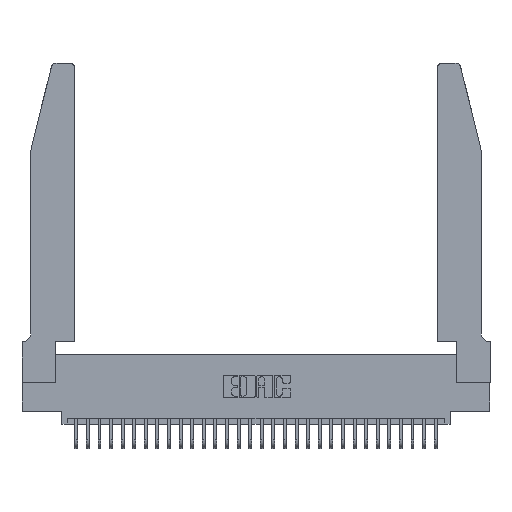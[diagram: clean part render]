
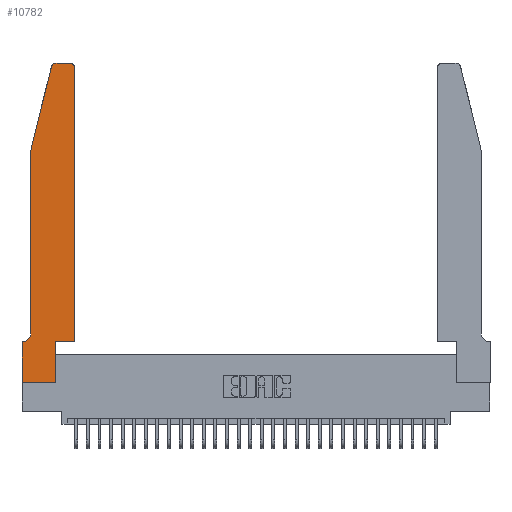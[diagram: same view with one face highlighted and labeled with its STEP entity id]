
A CAD part, top view. The second image highlights one B-rep face of the part: STEP entity #10782.
In plain terms, the highlighted planar face has unit normal (0, 0, 1).
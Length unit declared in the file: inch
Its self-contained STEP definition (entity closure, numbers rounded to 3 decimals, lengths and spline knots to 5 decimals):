
#184 = EDGE_CURVE ( 'NONE', #10911, #10960, #1109, .T. ) ;
#239 = VECTOR ( 'NONE', #18105, 39.37008 ) ;
#500 = CARTESIAN_POINT ( 'NONE',  ( 0.284, 2.75, 0.37 ) ) ;
#1109 = CIRCLE ( 'NONE', #26947, 0.07 ) ;
#1132 = CIRCLE ( 'NONE', #14062, 0.03 ) ;
#1803 = VERTEX_POINT ( 'NONE', #9535 ) ;
#2464 = VECTOR ( 'NONE', #32815, 39.37008 ) ;
#2518 = DIRECTION ( 'NONE',  ( 1., 0., 0. ) ) ;
#2710 = CARTESIAN_POINT ( 'NONE',  ( 0.4505, 0.35, 0.37 ) ) ;
#2935 = ORIENTED_EDGE ( 'NONE', *, *, #15527, .T. ) ;
#3083 = CIRCLE ( 'NONE', #22359, 0.03 ) ;
#3107 = VECTOR ( 'NONE', #7355, 39.37008 ) ;
#3114 = CARTESIAN_POINT ( 'NONE',  ( 0.0755, 0.35, 0.37 ) ) ;
#3702 = VERTEX_POINT ( 'NONE', #31811 ) ;
#4376 = ORIENTED_EDGE ( 'NONE', *, *, #26574, .T. ) ;
#4494 = VERTEX_POINT ( 'NONE', #19163 ) ;
#4568 = CARTESIAN_POINT ( 'NONE',  ( 0.0755, 2., 0.37 ) ) ;
#4871 = CARTESIAN_POINT ( 'NONE',  ( 0., 0., 0.37 ) ) ;
#4957 = CARTESIAN_POINT ( 'NONE',  ( 0.25487, 2.72718, 0.37 ) ) ;
#5204 = CARTESIAN_POINT ( 'NONE',  ( 0., 0.35, 0.37 ) ) ;
#5278 = DIRECTION ( 'NONE',  ( 0., 1., 0. ) ) ;
#5497 = DIRECTION ( 'NONE',  ( 0., 0., 1. ) ) ;
#5579 = ORIENTED_EDGE ( 'NONE', *, *, #6505, .T. ) ;
#6347 = DIRECTION ( 'NONE',  ( 1., 0., 0. ) ) ;
#6505 = EDGE_CURVE ( 'NONE', #4494, #7842, #20833, .T. ) ;
#6745 = EDGE_CURVE ( 'NONE', #9072, #10911, #13109, .T. ) ;
#7355 = DIRECTION ( 'NONE',  ( 1., 0., 0. ) ) ;
#7842 = VERTEX_POINT ( 'NONE', #19336 ) ;
#7913 = DIRECTION ( 'NONE',  ( 1., 0., 0. ) ) ;
#8019 = ORIENTED_EDGE ( 'NONE', *, *, #24753, .T. ) ;
#8052 = FACE_OUTER_BOUND ( 'NONE', #30361, .T. ) ;
#8519 = CARTESIAN_POINT ( 'NONE',  ( 0.0055, 0.35, 0.37 ) ) ;
#8548 = VERTEX_POINT ( 'NONE', #12256 ) ;
#9049 = ORIENTED_EDGE ( 'NONE', *, *, #23664, .T. ) ;
#9072 = VERTEX_POINT ( 'NONE', #14395 ) ;
#9352 = CARTESIAN_POINT ( 'NONE',  ( 0.0055, 0.42, 0.37 ) ) ;
#9535 = CARTESIAN_POINT ( 'NONE',  ( 0.4205, 2.75, 0.37 ) ) ;
#10027 = VECTOR ( 'NONE', #5278, 39.37008 ) ;
#10782 = ADVANCED_FACE ( 'NONE', ( #8052 ), #18148, .T. ) ;
#10911 = VERTEX_POINT ( 'NONE', #11079 ) ;
#10960 = VERTEX_POINT ( 'NONE', #8519 ) ;
#11079 = CARTESIAN_POINT ( 'NONE',  ( 0.0755, 0.42, 0.37 ) ) ;
#11301 = LINE ( 'NONE', #4568, #13681 ) ;
#11766 = CARTESIAN_POINT ( 'NONE',  ( 0.2865, 0.35, 0.37 ) ) ;
#12148 = DIRECTION ( 'NONE',  ( 0., 0., -1. ) ) ;
#12256 = CARTESIAN_POINT ( 'NONE',  ( 0.4505, 2.72, 0.37 ) ) ;
#12583 = LINE ( 'NONE', #27706, #16585 ) ;
#12739 = CARTESIAN_POINT ( 'NONE',  ( 0., 0., 0.37 ) ) ;
#13109 = LINE ( 'NONE', #29508, #22252 ) ;
#13526 = DIRECTION ( 'NONE',  ( 1., 0., 0. ) ) ;
#13681 = VECTOR ( 'NONE', #27495, 39.37008 ) ;
#14062 = AXIS2_PLACEMENT_3D ( 'NONE', #18311, #5497, #13526 ) ;
#14395 = CARTESIAN_POINT ( 'NONE',  ( 0.0755, 2., 0.37 ) ) ;
#15309 = VERTEX_POINT ( 'NONE', #25043 ) ;
#15527 = EDGE_CURVE ( 'NONE', #24561, #9072, #11301, .T. ) ;
#15559 = DIRECTION ( 'NONE',  ( -1., 0., 0. ) ) ;
#16585 = VECTOR ( 'NONE', #2518, 39.37008 ) ;
#16905 = ORIENTED_EDGE ( 'NONE', *, *, #6745, .T. ) ;
#17367 = DIRECTION ( 'NONE',  ( -1., 0., 0. ) ) ;
#17601 = VERTEX_POINT ( 'NONE', #12739 ) ;
#18105 = DIRECTION ( 'NONE',  ( -1., 0., 0. ) ) ;
#18148 = PLANE ( 'NONE',  #27326 ) ;
#18311 = CARTESIAN_POINT ( 'NONE',  ( 0.284, 2.72, 0.37 ) ) ;
#18360 = LINE ( 'NONE', #2710, #10027 ) ;
#18385 = DIRECTION ( 'NONE',  ( 0., -1., 0. ) ) ;
#19163 = CARTESIAN_POINT ( 'NONE',  ( 0.2865, 0., 0.37 ) ) ;
#19336 = CARTESIAN_POINT ( 'NONE',  ( 0.2865, 0.35, 0.37 ) ) ;
#19370 = ORIENTED_EDGE ( 'NONE', *, *, #31069, .T. ) ;
#20011 = VECTOR ( 'NONE', #15559, 39.37008 ) ;
#20019 = VECTOR ( 'NONE', #24338, 39.37008 ) ;
#20102 = ORIENTED_EDGE ( 'NONE', *, *, #184, .T. ) ;
#20575 = CARTESIAN_POINT ( 'NONE',  ( 0.2605, 2.75, 0.37 ) ) ;
#20833 = LINE ( 'NONE', #11766, #20019 ) ;
#21247 = ORIENTED_EDGE ( 'NONE', *, *, #25548, .T. ) ;
#22128 = ORIENTED_EDGE ( 'NONE', *, *, #28370, .T. ) ;
#22252 = VECTOR ( 'NONE', #18385, 39.37008 ) ;
#22359 = AXIS2_PLACEMENT_3D ( 'NONE', #26938, #29263, #6347 ) ;
#22439 = ORIENTED_EDGE ( 'NONE', *, *, #30471, .T. ) ;
#23123 = VERTEX_POINT ( 'NONE', #500 ) ;
#23132 = DIRECTION ( 'NONE',  ( 0., 0., 1. ) ) ;
#23664 = EDGE_CURVE ( 'NONE', #1803, #23123, #26328, .T. ) ;
#24338 = DIRECTION ( 'NONE',  ( 0., 1., 0. ) ) ;
#24561 = VERTEX_POINT ( 'NONE', #4957 ) ;
#24753 = EDGE_CURVE ( 'NONE', #23123, #24561, #1132, .T. ) ;
#25043 = CARTESIAN_POINT ( 'NONE',  ( 0., 0.35, 0.37 ) ) ;
#25548 = EDGE_CURVE ( 'NONE', #8548, #1803, #3083, .T. ) ;
#25791 = LINE ( 'NONE', #3114, #239 ) ;
#26328 = LINE ( 'NONE', #20575, #20011 ) ;
#26574 = EDGE_CURVE ( 'NONE', #10960, #15309, #25791, .T. ) ;
#26938 = CARTESIAN_POINT ( 'NONE',  ( 0.4205, 2.72, 0.37 ) ) ;
#26947 = AXIS2_PLACEMENT_3D ( 'NONE', #9352, #12148, #17367 ) ;
#27057 = LINE ( 'NONE', #30138, #3107 ) ;
#27326 = AXIS2_PLACEMENT_3D ( 'NONE', #5204, #23132, #7913 ) ;
#27495 = DIRECTION ( 'NONE',  ( -0.239, -0.971, 0. ) ) ;
#27706 = CARTESIAN_POINT ( 'NONE',  ( 0., 0., 0.37 ) ) ;
#28370 = EDGE_CURVE ( 'NONE', #17601, #4494, #12583, .T. ) ;
#29263 = DIRECTION ( 'NONE',  ( 0., 0., 1. ) ) ;
#29449 = ORIENTED_EDGE ( 'NONE', *, *, #32135, .T. ) ;
#29508 = CARTESIAN_POINT ( 'NONE',  ( 0.0755, 2., 0.37 ) ) ;
#30138 = CARTESIAN_POINT ( 'NONE',  ( 0.4505, 0.35, 0.37 ) ) ;
#30361 = EDGE_LOOP ( 'NONE', ( #9049, #8019, #2935, #16905, #20102, #4376, #22439, #22128, #5579, #29449, #19370, #21247 ) ) ;
#30471 = EDGE_CURVE ( 'NONE', #15309, #17601, #31118, .T. ) ;
#31069 = EDGE_CURVE ( 'NONE', #3702, #8548, #18360, .T. ) ;
#31118 = LINE ( 'NONE', #4871, #2464 ) ;
#31811 = CARTESIAN_POINT ( 'NONE',  ( 0.4505, 0.35, 0.37 ) ) ;
#32135 = EDGE_CURVE ( 'NONE', #7842, #3702, #27057, .T. ) ;
#32815 = DIRECTION ( 'NONE',  ( 0., -1., 0. ) ) ;
